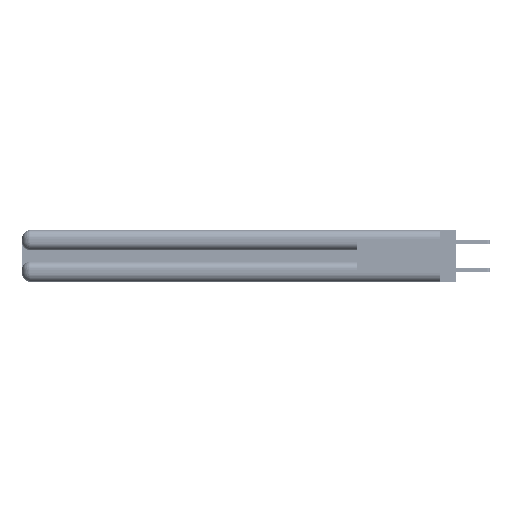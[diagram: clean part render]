
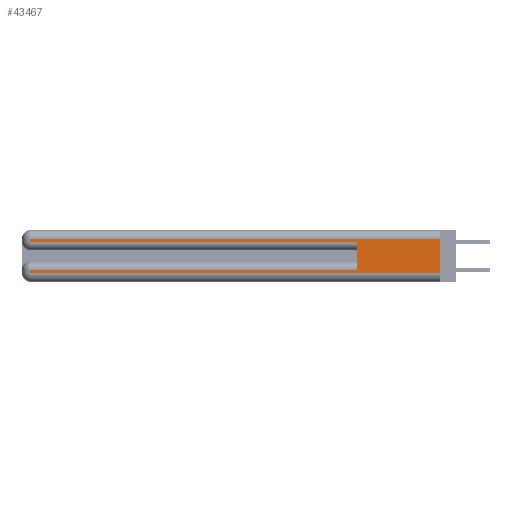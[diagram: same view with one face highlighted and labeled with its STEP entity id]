
A CAD part, left-side view. The second image highlights one B-rep face of the part: STEP entity #43467.
In plain terms, the highlighted planar face has unit normal (-1, 0, 0).
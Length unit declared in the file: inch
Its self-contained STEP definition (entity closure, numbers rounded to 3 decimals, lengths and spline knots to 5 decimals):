
#1271 = VERTEX_POINT ( 'NONE', #4625 ) ;
#1310 = CARTESIAN_POINT ( 'NONE',  ( 0., 2.94, 0.37 ) ) ;
#2773 = EDGE_CURVE ( 'NONE', #44468, #7109, #32843, .T. ) ;
#3210 = EDGE_CURVE ( 'NONE', #24606, #44468, #39247, .T. ) ;
#3661 = CARTESIAN_POINT ( 'NONE',  ( 0., 2.94, 0.31 ) ) ;
#3788 = EDGE_CURVE ( 'NONE', #24606, #44234, #44128, .T. ) ;
#4443 = EDGE_CURVE ( 'NONE', #1271, #35573, #35695, .T. ) ;
#4555 = CARTESIAN_POINT ( 'NONE',  ( 0., 0.6, 0.285 ) ) ;
#4625 = CARTESIAN_POINT ( 'NONE',  ( 0., 2.94, 0.085 ) ) ;
#5287 = ORIENTED_EDGE ( 'NONE', *, *, #15541, .F. ) ;
#6795 = VECTOR ( 'NONE', #43252, 39.37008 ) ;
#7109 = VERTEX_POINT ( 'NONE', #14554 ) ;
#7164 = LINE ( 'NONE', #20800, #24464 ) ;
#7568 = VECTOR ( 'NONE', #11178, 39.37008 ) ;
#7800 = ORIENTED_EDGE ( 'NONE', *, *, #30411, .T. ) ;
#7971 = VECTOR ( 'NONE', #43145, 39.37008 ) ;
#9779 = CARTESIAN_POINT ( 'NONE',  ( 0., 0., 0.085 ) ) ;
#11178 = DIRECTION ( 'NONE',  ( 0., 0., -1. ) ) ;
#12589 = CARTESIAN_POINT ( 'NONE',  ( 0., 0.6, 0.145 ) ) ;
#13043 = VECTOR ( 'NONE', #30745, 39.37008 ) ;
#13271 = DIRECTION ( 'NONE',  ( 0., -1., 0. ) ) ;
#14458 = VECTOR ( 'NONE', #21843, 39.37008 ) ;
#14554 = CARTESIAN_POINT ( 'NONE',  ( 0., 2.94, 0.285 ) ) ;
#14781 = ORIENTED_EDGE ( 'NONE', *, *, #4443, .T. ) ;
#14784 = CARTESIAN_POINT ( 'NONE',  ( 0., 2.94, 0.06 ) ) ;
#15027 = ORIENTED_EDGE ( 'NONE', *, *, #3210, .T. ) ;
#15541 = EDGE_CURVE ( 'NONE', #33662, #20868, #33740, .T. ) ;
#15700 = DIRECTION ( 'NONE',  ( 0., 1., 0. ) ) ;
#17163 = VECTOR ( 'NONE', #15700, 39.37008 ) ;
#17998 = CARTESIAN_POINT ( 'NONE',  ( 0., 0., 0.31 ) ) ;
#18527 = CARTESIAN_POINT ( 'NONE',  ( 0., 0., 0.06 ) ) ;
#18585 = DIRECTION ( 'NONE',  ( 1., 0., 0. ) ) ;
#18638 = VECTOR ( 'NONE', #37203, 39.37008 ) ;
#19961 = EDGE_CURVE ( 'NONE', #33662, #1271, #31405, .T. ) ;
#20800 = CARTESIAN_POINT ( 'NONE',  ( 0., 0., 0.06 ) ) ;
#20868 = VERTEX_POINT ( 'NONE', #4555 ) ;
#21843 = DIRECTION ( 'NONE',  ( 0., 0., -1. ) ) ;
#22910 = EDGE_LOOP ( 'NONE', ( #30200, #15027, #22933, #7800, #5287, #23944, #14781, #43592 ) ) ;
#22933 = ORIENTED_EDGE ( 'NONE', *, *, #2773, .T. ) ;
#23385 = AXIS2_PLACEMENT_3D ( 'NONE', #28501, #18585, #28809 ) ;
#23629 = CARTESIAN_POINT ( 'NONE',  ( 0., 0.6, 0.085 ) ) ;
#23944 = ORIENTED_EDGE ( 'NONE', *, *, #19961, .T. ) ;
#24464 = VECTOR ( 'NONE', #13271, 39.37008 ) ;
#24606 = VERTEX_POINT ( 'NONE', #17998 ) ;
#27422 = EDGE_CURVE ( 'NONE', #35573, #44234, #7164, .T. ) ;
#28501 = CARTESIAN_POINT ( 'NONE',  ( 0., 0., 0.37 ) ) ;
#28809 = DIRECTION ( 'NONE',  ( 0., 0., -1. ) ) ;
#29108 = CARTESIAN_POINT ( 'NONE',  ( 0., 0., 0.31 ) ) ;
#29581 = CARTESIAN_POINT ( 'NONE',  ( 0., 0., 0.285 ) ) ;
#30200 = ORIENTED_EDGE ( 'NONE', *, *, #3788, .F. ) ;
#30411 = EDGE_CURVE ( 'NONE', #7109, #20868, #32803, .T. ) ;
#30745 = DIRECTION ( 'NONE',  ( 0., 1., 0. ) ) ;
#31405 = LINE ( 'NONE', #9779, #13043 ) ;
#32803 = LINE ( 'NONE', #29581, #7971 ) ;
#32843 = LINE ( 'NONE', #1310, #14458 ) ;
#32871 = FACE_OUTER_BOUND ( 'NONE', #22910, .T. ) ;
#33662 = VERTEX_POINT ( 'NONE', #23629 ) ;
#33740 = LINE ( 'NONE', #12589, #18638 ) ;
#34750 = CARTESIAN_POINT ( 'NONE',  ( 0., 2.94, 0.37 ) ) ;
#35552 = CARTESIAN_POINT ( 'NONE',  ( 0., 0., 0.37 ) ) ;
#35573 = VERTEX_POINT ( 'NONE', #14784 ) ;
#35695 = LINE ( 'NONE', #34750, #7568 ) ;
#37203 = DIRECTION ( 'NONE',  ( 0., 0., 1. ) ) ;
#38924 = PLANE ( 'NONE',  #23385 ) ;
#39247 = LINE ( 'NONE', #29108, #17163 ) ;
#43145 = DIRECTION ( 'NONE',  ( 0., -1., 0. ) ) ;
#43252 = DIRECTION ( 'NONE',  ( 0., 0., -1. ) ) ;
#43467 = ADVANCED_FACE ( 'NONE', ( #32871 ), #38924, .F. ) ;
#43592 = ORIENTED_EDGE ( 'NONE', *, *, #27422, .T. ) ;
#44128 = LINE ( 'NONE', #35552, #6795 ) ;
#44234 = VERTEX_POINT ( 'NONE', #18527 ) ;
#44468 = VERTEX_POINT ( 'NONE', #3661 ) ;
